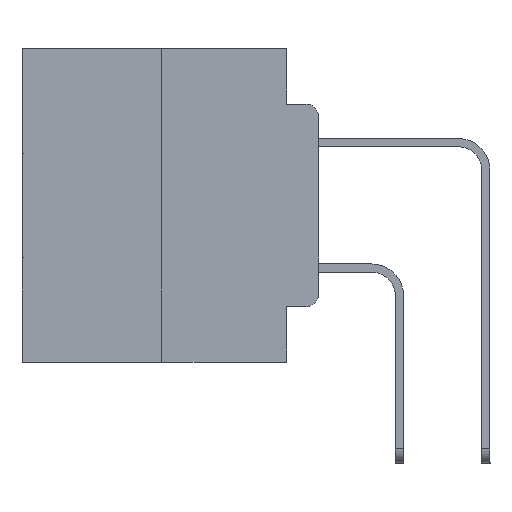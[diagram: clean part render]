
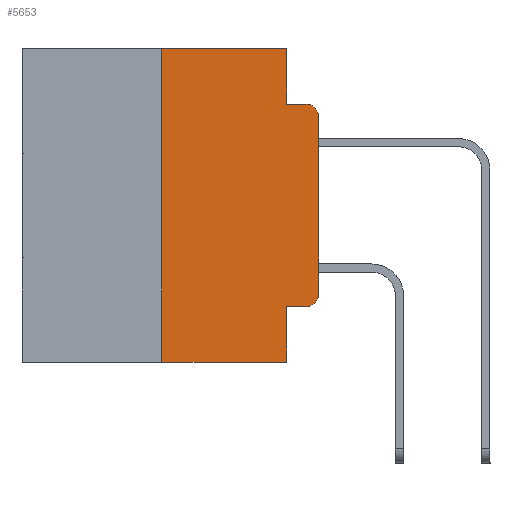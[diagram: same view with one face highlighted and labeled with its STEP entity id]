
A CAD part, left-side view. The second image highlights one B-rep face of the part: STEP entity #5653.
In plain terms, the highlighted planar face has unit normal (-1, 0, 0).
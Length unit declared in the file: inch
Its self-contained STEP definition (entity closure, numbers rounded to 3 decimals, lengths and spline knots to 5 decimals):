
#287 = EDGE_CURVE ( 'NONE', #19100, #5506, #2507, .T. ) ;
#469 = EDGE_CURVE ( 'NONE', #4006, #2431, #4387, .T. ) ;
#682 = ORIENTED_EDGE ( 'NONE', *, *, #27846, .F. ) ;
#1624 = LINE ( 'NONE', #16281, #26326 ) ;
#1884 = CIRCLE ( 'NONE', #6030, 0.02 ) ;
#2154 = VECTOR ( 'NONE', #10295, 39.37008 ) ;
#2207 = LINE ( 'NONE', #15849, #8449 ) ;
#2431 = VERTEX_POINT ( 'NONE', #21210 ) ;
#2491 = ORIENTED_EDGE ( 'NONE', *, *, #8747, .T. ) ;
#2507 = LINE ( 'NONE', #17323, #21058 ) ;
#3215 = DIRECTION ( 'NONE',  ( 1., 0., 0. ) ) ;
#3677 = LINE ( 'NONE', #4614, #16017 ) ;
#4006 = VERTEX_POINT ( 'NONE', #5216 ) ;
#4013 = VECTOR ( 'NONE', #16103, 39.37008 ) ;
#4376 = ORIENTED_EDGE ( 'NONE', *, *, #21852, .F. ) ;
#4387 = LINE ( 'NONE', #6683, #21848 ) ;
#4614 = CARTESIAN_POINT ( 'NONE',  ( 0., 0.051, -0.0885 ) ) ;
#5216 = CARTESIAN_POINT ( 'NONE',  ( 0., 0.051, -0.4115 ) ) ;
#5394 = CARTESIAN_POINT ( 'NONE',  ( 0., 0.051, -0.5 ) ) ;
#5506 = VERTEX_POINT ( 'NONE', #23385 ) ;
#5653 = ADVANCED_FACE ( 'NONE', ( #15502 ), #26194, .F. ) ;
#6030 = AXIS2_PLACEMENT_3D ( 'NONE', #27752, #13978, #10299 ) ;
#6683 = CARTESIAN_POINT ( 'NONE',  ( 0., 0.051, -0.4115 ) ) ;
#7299 = VERTEX_POINT ( 'NONE', #16459 ) ;
#7658 = ORIENTED_EDGE ( 'NONE', *, *, #287, .T. ) ;
#7741 = CARTESIAN_POINT ( 'NONE',  ( 0., 0.473, 0. ) ) ;
#7975 = CARTESIAN_POINT ( 'NONE',  ( 0., 0.25, 0. ) ) ;
#8449 = VECTOR ( 'NONE', #11236, 39.37008 ) ;
#8485 = CARTESIAN_POINT ( 'NONE',  ( 0., 0., -0.3915 ) ) ;
#8747 = EDGE_CURVE ( 'NONE', #5506, #8843, #16027, .T. ) ;
#8843 = VERTEX_POINT ( 'NONE', #20785 ) ;
#10295 = DIRECTION ( 'NONE',  ( 0., 0., 1. ) ) ;
#10299 = DIRECTION ( 'NONE',  ( 0., 0., -1. ) ) ;
#10422 = DIRECTION ( 'NONE',  ( 0., -1., 0. ) ) ;
#11103 = DIRECTION ( 'NONE',  ( 0., -1., 0. ) ) ;
#11236 = DIRECTION ( 'NONE',  ( 0., 0., -1. ) ) ;
#11361 = AXIS2_PLACEMENT_3D ( 'NONE', #7741, #3215, #19467 ) ;
#11429 = EDGE_CURVE ( 'NONE', #4006, #24590, #2207, .T. ) ;
#11934 = ORIENTED_EDGE ( 'NONE', *, *, #469, .T. ) ;
#12852 = CARTESIAN_POINT ( 'NONE',  ( 0., 0.25, -0.5 ) ) ;
#12985 = EDGE_CURVE ( 'NONE', #13724, #20239, #20728, .T. ) ;
#13367 = VERTEX_POINT ( 'NONE', #25422 ) ;
#13568 = DIRECTION ( 'NONE',  ( -1., 0., 0. ) ) ;
#13724 = VERTEX_POINT ( 'NONE', #12852 ) ;
#13978 = DIRECTION ( 'NONE',  ( -1., 0., 0. ) ) ;
#15502 = FACE_OUTER_BOUND ( 'NONE', #23349, .T. ) ;
#15849 = CARTESIAN_POINT ( 'NONE',  ( 0., 0.051, 0. ) ) ;
#16017 = VECTOR ( 'NONE', #20793, 39.37008 ) ;
#16027 = CIRCLE ( 'NONE', #19618, 0.02 ) ;
#16103 = DIRECTION ( 'NONE',  ( 0., -1., 0. ) ) ;
#16281 = CARTESIAN_POINT ( 'NONE',  ( 0., 0.051, 0. ) ) ;
#16459 = CARTESIAN_POINT ( 'NONE',  ( 0., 0.051, 0. ) ) ;
#16704 = ORIENTED_EDGE ( 'NONE', *, *, #28466, .T. ) ;
#17232 = DIRECTION ( 'NONE',  ( 0., 0., 1. ) ) ;
#17323 = CARTESIAN_POINT ( 'NONE',  ( 0., 0., 0. ) ) ;
#19100 = VERTEX_POINT ( 'NONE', #8485 ) ;
#19467 = DIRECTION ( 'NONE',  ( 0., 0., -1. ) ) ;
#19618 = AXIS2_PLACEMENT_3D ( 'NONE', #27351, #13568, #29600 ) ;
#20239 = VERTEX_POINT ( 'NONE', #25875 ) ;
#20728 = LINE ( 'NONE', #7975, #2154 ) ;
#20785 = CARTESIAN_POINT ( 'NONE',  ( 0., 0.02, -0.0885 ) ) ;
#20793 = DIRECTION ( 'NONE',  ( 0., -1., 0. ) ) ;
#20797 = EDGE_CURVE ( 'NONE', #7299, #13367, #1624, .T. ) ;
#21058 = VECTOR ( 'NONE', #17232, 39.37008 ) ;
#21210 = CARTESIAN_POINT ( 'NONE',  ( 0., 0.02, -0.4115 ) ) ;
#21848 = VECTOR ( 'NONE', #10422, 39.37008 ) ;
#21852 = EDGE_CURVE ( 'NONE', #20239, #7299, #28716, .T. ) ;
#22494 = LINE ( 'NONE', #27523, #4013 ) ;
#23086 = ORIENTED_EDGE ( 'NONE', *, *, #25967, .T. ) ;
#23349 = EDGE_LOOP ( 'NONE', ( #7658, #2491, #682, #29870, #4376, #26007, #16704, #24250, #11934, #23086 ) ) ;
#23385 = CARTESIAN_POINT ( 'NONE',  ( 0., 0., -0.1085 ) ) ;
#23390 = VECTOR ( 'NONE', #11103, 39.37008 ) ;
#24250 = ORIENTED_EDGE ( 'NONE', *, *, #11429, .F. ) ;
#24590 = VERTEX_POINT ( 'NONE', #5394 ) ;
#25422 = CARTESIAN_POINT ( 'NONE',  ( 0., 0.051, -0.0885 ) ) ;
#25875 = CARTESIAN_POINT ( 'NONE',  ( 0., 0.25, 0. ) ) ;
#25967 = EDGE_CURVE ( 'NONE', #2431, #19100, #1884, .T. ) ;
#26007 = ORIENTED_EDGE ( 'NONE', *, *, #12985, .F. ) ;
#26194 = PLANE ( 'NONE',  #11361 ) ;
#26326 = VECTOR ( 'NONE', #29946, 39.37008 ) ;
#27251 = CARTESIAN_POINT ( 'NONE',  ( 0., 0.473, 0. ) ) ;
#27351 = CARTESIAN_POINT ( 'NONE',  ( 0., 0.02, -0.1085 ) ) ;
#27523 = CARTESIAN_POINT ( 'NONE',  ( 0., 0.473, -0.5 ) ) ;
#27752 = CARTESIAN_POINT ( 'NONE',  ( 0., 0.02, -0.3915 ) ) ;
#27846 = EDGE_CURVE ( 'NONE', #13367, #8843, #3677, .T. ) ;
#28466 = EDGE_CURVE ( 'NONE', #13724, #24590, #22494, .T. ) ;
#28716 = LINE ( 'NONE', #27251, #23390 ) ;
#29600 = DIRECTION ( 'NONE',  ( 0., 0., -1. ) ) ;
#29870 = ORIENTED_EDGE ( 'NONE', *, *, #20797, .F. ) ;
#29946 = DIRECTION ( 'NONE',  ( 0., 0., -1. ) ) ;
